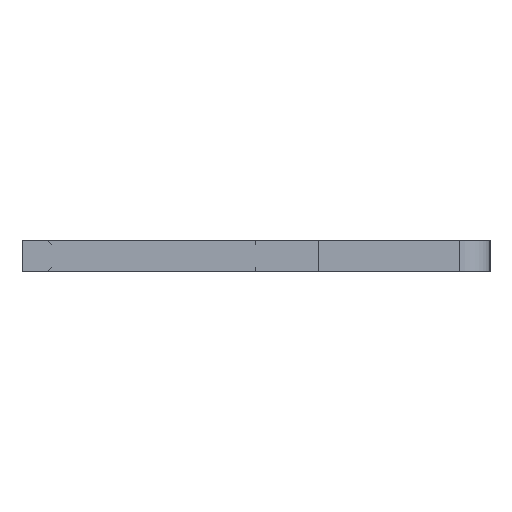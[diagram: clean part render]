
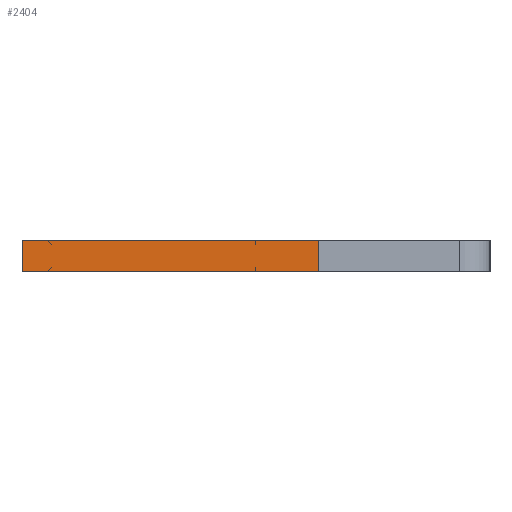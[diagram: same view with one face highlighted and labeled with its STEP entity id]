
A CAD part, left-side view. The second image highlights one B-rep face of the part: STEP entity #2404.
In plain terms, the highlighted face is planar.
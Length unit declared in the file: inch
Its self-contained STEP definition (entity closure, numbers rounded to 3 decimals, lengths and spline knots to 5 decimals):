
#84 = LINE ( 'NONE', #251, #2885 ) ;
#132 = VERTEX_POINT ( 'NONE', #1597 ) ;
#162 = EDGE_CURVE ( 'NONE', #3366, #132, #2595, .T. ) ;
#180 = PLANE ( 'NONE',  #1976 ) ;
#251 = CARTESIAN_POINT ( 'NONE',  ( 0.01, -0.04, -0.04 ) ) ;
#433 = ORIENTED_EDGE ( 'NONE', *, *, #3209, .T. ) ;
#476 = DIRECTION ( 'NONE',  ( 0., 1., 0. ) ) ;
#480 = VECTOR ( 'NONE', #1076, 39.37008 ) ;
#538 = CARTESIAN_POINT ( 'NONE',  ( 0.01, 0.15, -0.04 ) ) ;
#560 = VECTOR ( 'NONE', #476, 39.37008 ) ;
#643 = FACE_OUTER_BOUND ( 'NONE', #938, .T. ) ;
#672 = CARTESIAN_POINT ( 'NONE',  ( -0.01, -0.04, -0.04 ) ) ;
#794 = CARTESIAN_POINT ( 'NONE',  ( 0.01, -0.04, -0.04 ) ) ;
#938 = EDGE_LOOP ( 'NONE', ( #3106, #3360, #1711, #433 ) ) ;
#1039 = DIRECTION ( 'NONE',  ( -1., 0., 0. ) ) ;
#1076 = DIRECTION ( 'NONE',  ( 0., 1., 0. ) ) ;
#1597 = CARTESIAN_POINT ( 'NONE',  ( 0.01, 0.15, -0.04 ) ) ;
#1711 = ORIENTED_EDGE ( 'NONE', *, *, #162, .F. ) ;
#1877 = VERTEX_POINT ( 'NONE', #672 ) ;
#1976 = AXIS2_PLACEMENT_3D ( 'NONE', #3433, #2878, #2892 ) ;
#1991 = CARTESIAN_POINT ( 'NONE',  ( -0.01, 0.15, -0.04 ) ) ;
#1993 = LINE ( 'NONE', #538, #2420 ) ;
#2081 = VERTEX_POINT ( 'NONE', #1991 ) ;
#2128 = CARTESIAN_POINT ( 'NONE',  ( 0.01, 0.15, -0.04 ) ) ;
#2404 = ADVANCED_FACE ( 'NONE', ( #643 ), #180, .F. ) ;
#2420 = VECTOR ( 'NONE', #2430, 39.37008 ) ;
#2430 = DIRECTION ( 'NONE',  ( -1., 0., 0. ) ) ;
#2595 = LINE ( 'NONE', #2128, #480 ) ;
#2878 = DIRECTION ( 'NONE',  ( 0., 0., 1. ) ) ;
#2885 = VECTOR ( 'NONE', #1039, 39.37008 ) ;
#2892 = DIRECTION ( 'NONE',  ( 1., 0., 0. ) ) ;
#2953 = EDGE_CURVE ( 'NONE', #1877, #2081, #3317, .T. ) ;
#3106 = ORIENTED_EDGE ( 'NONE', *, *, #2953, .T. ) ;
#3160 = EDGE_CURVE ( 'NONE', #132, #2081, #1993, .T. ) ;
#3209 = EDGE_CURVE ( 'NONE', #3366, #1877, #84, .T. ) ;
#3242 = CARTESIAN_POINT ( 'NONE',  ( -0.01, 0.15, -0.04 ) ) ;
#3317 = LINE ( 'NONE', #3242, #560 ) ;
#3360 = ORIENTED_EDGE ( 'NONE', *, *, #3160, .F. ) ;
#3366 = VERTEX_POINT ( 'NONE', #794 ) ;
#3433 = CARTESIAN_POINT ( 'NONE',  ( 0.01, 0.15, -0.04 ) ) ;
